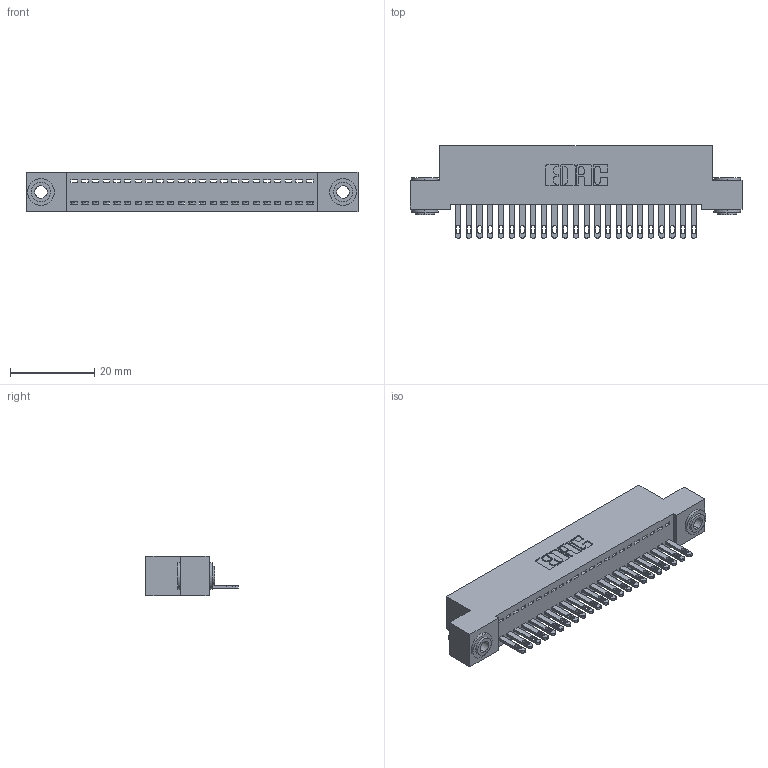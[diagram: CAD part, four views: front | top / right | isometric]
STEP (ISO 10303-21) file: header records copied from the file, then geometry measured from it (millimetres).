
FILE_DESCRIPTION (( 'STEP AP203' ), '1' );
FILE_NAME ('342-023-500-103.STEP', '2018-08-11T01:17:05', ( '' ), ( '' ), 'SwSTEP 2.0', 'SolidWorks 2016', '' );
FILE_SCHEMA (( 'CONFIG_CONTROL_DESIGN' ));
Length unit declared in the file: inch
Products named in the file (4): 342-023-500-103; 342 Part_.156 TH; 345-292-001_345-293-100; 342-250-002_345-250-002-102
Assembly tree (26 placements, depth 2):
  342-023-500-103
    342 Part_.156 TH
    345-292-001_345-293-100  x23
    342-250-002_345-250-002-102  x2
Bounding box: 78.74 x 21.85 x 9.4 mm (x, y, z)
Volume: 6871 mm3; surface area: 10006.4 mm2
Topology: 26 solids, 26 shells, 1390 faces, 4239 edges, 2822 vertices
Faces by surface type: plane 904, cylinder 478, cone 8
Entity records: 16966 total; most frequent: CARTESIAN_POINT 2906, ORIENTED_EDGE 2858, DIRECTION 2525, EDGE_CURVE 1429, VECTOR 1273, LINE 1273, VERTEX_POINT 950, AXIS2_PLACEMENT_3D 626
